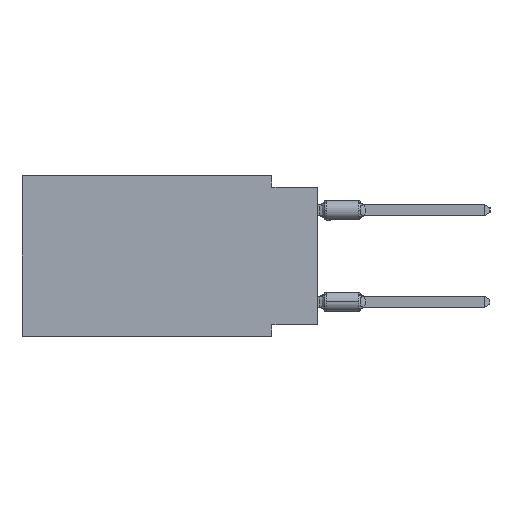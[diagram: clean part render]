
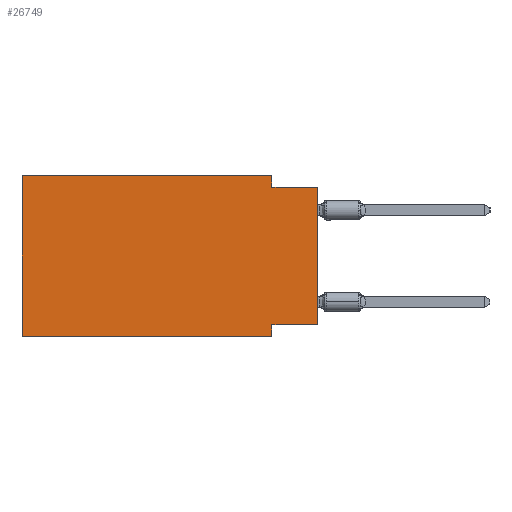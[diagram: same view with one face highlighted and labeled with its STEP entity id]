
A CAD part, left-side view. The second image highlights one B-rep face of the part: STEP entity #26749.
In plain terms, the highlighted planar face has unit normal (-1, 0, 0).
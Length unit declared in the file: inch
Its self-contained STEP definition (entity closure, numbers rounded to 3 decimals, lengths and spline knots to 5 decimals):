
#1379 = CARTESIAN_POINT ( 'NONE',  ( 0., 0.1, 0. ) ) ;
#2643 = DIRECTION ( 'NONE',  ( 0., 1., 0. ) ) ;
#2691 = CARTESIAN_POINT ( 'NONE',  ( 0., 0.645, -0.35 ) ) ;
#3622 = EDGE_CURVE ( 'NONE', #9502, #25057, #25763, .T. ) ;
#3918 = VECTOR ( 'NONE', #48543, 39.37008 ) ;
#4202 = VECTOR ( 'NONE', #2643, 39.37008 ) ;
#4490 = CARTESIAN_POINT ( 'NONE',  ( 0., 0., 0. ) ) ;
#5071 = VERTEX_POINT ( 'NONE', #2691 ) ;
#5565 = LINE ( 'NONE', #1379, #54131 ) ;
#5593 = ORIENTED_EDGE ( 'NONE', *, *, #3622, .F. ) ;
#7274 = AXIS2_PLACEMENT_3D ( 'NONE', #7804, #34254, #48084 ) ;
#7804 = CARTESIAN_POINT ( 'NONE',  ( 0., 0.645, 0. ) ) ;
#7847 = VECTOR ( 'NONE', #38628, 39.37008 ) ;
#8837 = LINE ( 'NONE', #54845, #29547 ) ;
#9502 = VERTEX_POINT ( 'NONE', #39707 ) ;
#10426 = EDGE_CURVE ( 'NONE', #25057, #57605, #57279, .T. ) ;
#11413 = CARTESIAN_POINT ( 'NONE',  ( 0., 0.1, -0.325 ) ) ;
#13611 = DIRECTION ( 'NONE',  ( 0., -1., 0. ) ) ;
#13812 = DIRECTION ( 'NONE',  ( 0., 0., 1. ) ) ;
#15091 = VERTEX_POINT ( 'NONE', #28716 ) ;
#15837 = EDGE_LOOP ( 'NONE', ( #37284, #22450, #33042, #45529, #55462, #23821, #23929, #5593 ) ) ;
#16661 = CARTESIAN_POINT ( 'NONE',  ( 0., 0.1, -0.35 ) ) ;
#17678 = EDGE_CURVE ( 'NONE', #22260, #15091, #34707, .T. ) ;
#17702 = CARTESIAN_POINT ( 'NONE',  ( 0., 0.1, -0.025 ) ) ;
#21329 = PLANE ( 'NONE',  #7274 ) ;
#21910 = VECTOR ( 'NONE', #13611, 39.37008 ) ;
#22260 = VERTEX_POINT ( 'NONE', #37132 ) ;
#22450 = ORIENTED_EDGE ( 'NONE', *, *, #53633, .F. ) ;
#23735 = EDGE_CURVE ( 'NONE', #9502, #49547, #46563, .T. ) ;
#23818 = CARTESIAN_POINT ( 'NONE',  ( 0., 0.645, -0.35 ) ) ;
#23821 = ORIENTED_EDGE ( 'NONE', *, *, #31074, .T. ) ;
#23929 = ORIENTED_EDGE ( 'NONE', *, *, #10426, .F. ) ;
#24663 = CARTESIAN_POINT ( 'NONE',  ( 0., 0.1, -0.35 ) ) ;
#25057 = VERTEX_POINT ( 'NONE', #11413 ) ;
#25763 = LINE ( 'NONE', #43796, #4202 ) ;
#26404 = VERTEX_POINT ( 'NONE', #17702 ) ;
#26749 = ADVANCED_FACE ( 'NONE', ( #35427 ), #21329, .F. ) ;
#28716 = CARTESIAN_POINT ( 'NONE',  ( 0., 0.1, 0. ) ) ;
#29547 = VECTOR ( 'NONE', #55746, 39.37008 ) ;
#29857 = DIRECTION ( 'NONE',  ( 0., 0., -1. ) ) ;
#31074 = EDGE_CURVE ( 'NONE', #5071, #57605, #55715, .T. ) ;
#32616 = CARTESIAN_POINT ( 'NONE',  ( 0., 0., -0.025 ) ) ;
#33042 = ORIENTED_EDGE ( 'NONE', *, *, #34226, .F. ) ;
#34226 = EDGE_CURVE ( 'NONE', #15091, #26404, #5565, .T. ) ;
#34254 = DIRECTION ( 'NONE',  ( 1., 0., 0. ) ) ;
#34676 = CARTESIAN_POINT ( 'NONE',  ( 0., 0., -0.025 ) ) ;
#34707 = LINE ( 'NONE', #48570, #7847 ) ;
#35427 = FACE_OUTER_BOUND ( 'NONE', #15837, .T. ) ;
#37132 = CARTESIAN_POINT ( 'NONE',  ( 0., 0.645, 0. ) ) ;
#37284 = ORIENTED_EDGE ( 'NONE', *, *, #23735, .T. ) ;
#38628 = DIRECTION ( 'NONE',  ( 0., -1., 0. ) ) ;
#38964 = EDGE_CURVE ( 'NONE', #5071, #22260, #8837, .T. ) ;
#39707 = CARTESIAN_POINT ( 'NONE',  ( 0., 0., -0.325 ) ) ;
#42825 = VECTOR ( 'NONE', #13812, 39.37008 ) ;
#43796 = CARTESIAN_POINT ( 'NONE',  ( 0., 0., -0.325 ) ) ;
#45529 = ORIENTED_EDGE ( 'NONE', *, *, #17678, .F. ) ;
#46563 = LINE ( 'NONE', #4490, #42825 ) ;
#48084 = DIRECTION ( 'NONE',  ( 0., 0., -1. ) ) ;
#48543 = DIRECTION ( 'NONE',  ( 0., -1., 0. ) ) ;
#48570 = CARTESIAN_POINT ( 'NONE',  ( 0., 0.645, 0. ) ) ;
#49547 = VERTEX_POINT ( 'NONE', #32616 ) ;
#51567 = DIRECTION ( 'NONE',  ( 0., 0., -1. ) ) ;
#52064 = VECTOR ( 'NONE', #29857, 39.37008 ) ;
#53633 = EDGE_CURVE ( 'NONE', #26404, #49547, #56992, .T. ) ;
#54131 = VECTOR ( 'NONE', #51567, 39.37008 ) ;
#54845 = CARTESIAN_POINT ( 'NONE',  ( 0., 0.645, 0. ) ) ;
#55462 = ORIENTED_EDGE ( 'NONE', *, *, #38964, .F. ) ;
#55715 = LINE ( 'NONE', #23818, #21910 ) ;
#55746 = DIRECTION ( 'NONE',  ( 0., 0., 1. ) ) ;
#56992 = LINE ( 'NONE', #34676, #3918 ) ;
#57279 = LINE ( 'NONE', #16661, #52064 ) ;
#57605 = VERTEX_POINT ( 'NONE', #24663 ) ;
